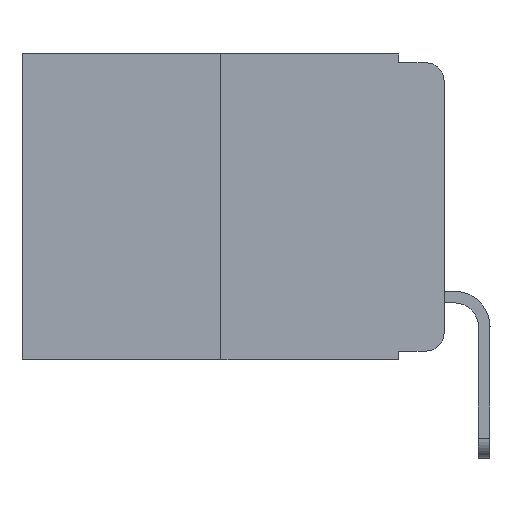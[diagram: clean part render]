
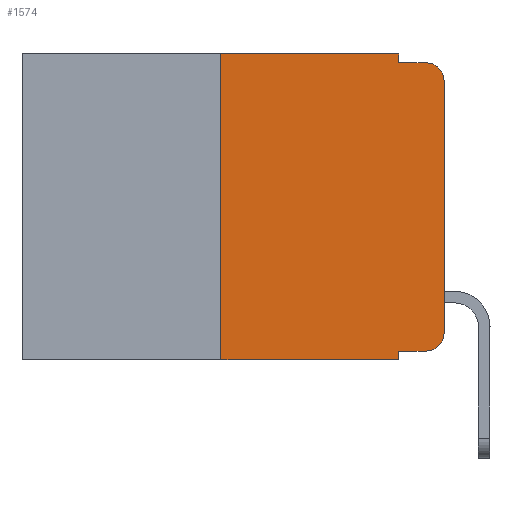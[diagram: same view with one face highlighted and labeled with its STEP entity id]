
A CAD part, left-side view. The second image highlights one B-rep face of the part: STEP entity #1574.
In plain terms, the highlighted planar face has unit normal (-1, 0, 0).
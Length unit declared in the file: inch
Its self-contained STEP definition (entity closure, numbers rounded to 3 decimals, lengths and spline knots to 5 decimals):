
#484 = CARTESIAN_POINT ( 'NONE',  ( 0., 0.25, 0. ) ) ;
#610 = EDGE_LOOP ( 'NONE', ( #824, #9862, #5833, #13297, #13022, #4682, #11914, #13391, #3550, #8004 ) ) ;
#616 = CARTESIAN_POINT ( 'NONE',  ( 0., 0., -0.313 ) ) ;
#824 = ORIENTED_EDGE ( 'NONE', *, *, #12422, .T. ) ;
#927 = VERTEX_POINT ( 'NONE', #6848 ) ;
#1211 = LINE ( 'NONE', #8619, #12267 ) ;
#1288 = EDGE_CURVE ( 'NONE', #4312, #3890, #7972, .T. ) ;
#1327 = DIRECTION ( 'NONE',  ( 0., -1., 0. ) ) ;
#1410 = CARTESIAN_POINT ( 'NONE',  ( 0., 0.051, -0.01 ) ) ;
#1574 = ADVANCED_FACE ( 'NONE', ( #6616 ), #6481, .F. ) ;
#1630 = DIRECTION ( 'NONE',  ( 0., -1., 0. ) ) ;
#1745 = DIRECTION ( 'NONE',  ( 0., -1., 0. ) ) ;
#2268 = DIRECTION ( 'NONE',  ( -1., 0., 0. ) ) ;
#2373 = VERTEX_POINT ( 'NONE', #616 ) ;
#2387 = LINE ( 'NONE', #8797, #4918 ) ;
#2411 = AXIS2_PLACEMENT_3D ( 'NONE', #8838, #7982, #7907 ) ;
#2805 = AXIS2_PLACEMENT_3D ( 'NONE', #11818, #2268, #8746 ) ;
#2826 = CARTESIAN_POINT ( 'NONE',  ( 0., 0.473, 0. ) ) ;
#2977 = VECTOR ( 'NONE', #11652, 39.37008 ) ;
#3105 = LINE ( 'NONE', #11745, #5889 ) ;
#3157 = VERTEX_POINT ( 'NONE', #8513 ) ;
#3550 = ORIENTED_EDGE ( 'NONE', *, *, #8214, .T. ) ;
#3738 = EDGE_CURVE ( 'NONE', #6555, #2373, #12442, .T. ) ;
#3823 = LINE ( 'NONE', #8264, #9161 ) ;
#3890 = VERTEX_POINT ( 'NONE', #7125 ) ;
#4067 = CARTESIAN_POINT ( 'NONE',  ( 0., 0., -0.03 ) ) ;
#4140 = EDGE_CURVE ( 'NONE', #7694, #6399, #5588, .T. ) ;
#4312 = VERTEX_POINT ( 'NONE', #4067 ) ;
#4591 = DIRECTION ( 'NONE',  ( 0., 0., 1. ) ) ;
#4682 = ORIENTED_EDGE ( 'NONE', *, *, #4140, .F. ) ;
#4714 = VECTOR ( 'NONE', #1745, 39.37008 ) ;
#4891 = DIRECTION ( 'NONE',  ( 0., 0., -1. ) ) ;
#4918 = VECTOR ( 'NONE', #1327, 39.37008 ) ;
#5342 = LINE ( 'NONE', #8439, #2977 ) ;
#5368 = CARTESIAN_POINT ( 'NONE',  ( 0., 0.02, -0.333 ) ) ;
#5435 = DIRECTION ( 'NONE',  ( 1., 0., 0. ) ) ;
#5523 = DIRECTION ( 'NONE',  ( 0., 0., -1. ) ) ;
#5588 = LINE ( 'NONE', #484, #13322 ) ;
#5833 = ORIENTED_EDGE ( 'NONE', *, *, #10413, .F. ) ;
#5889 = VECTOR ( 'NONE', #7387, 39.37008 ) ;
#5971 = EDGE_CURVE ( 'NONE', #3157, #12062, #3823, .T. ) ;
#6377 = VERTEX_POINT ( 'NONE', #1410 ) ;
#6399 = VERTEX_POINT ( 'NONE', #12319 ) ;
#6410 = CARTESIAN_POINT ( 'NONE',  ( 0., 0.051, -0.343 ) ) ;
#6416 = DIRECTION ( 'NONE',  ( 0., 0., -1. ) ) ;
#6481 = PLANE ( 'NONE',  #7869 ) ;
#6555 = VERTEX_POINT ( 'NONE', #5368 ) ;
#6616 = FACE_OUTER_BOUND ( 'NONE', #610, .T. ) ;
#6716 = EDGE_CURVE ( 'NONE', #7694, #12062, #2387, .T. ) ;
#6848 = CARTESIAN_POINT ( 'NONE',  ( 0., 0.051, 0. ) ) ;
#7046 = LINE ( 'NONE', #2826, #13811 ) ;
#7125 = CARTESIAN_POINT ( 'NONE',  ( 0., 0.02, -0.01 ) ) ;
#7387 = DIRECTION ( 'NONE',  ( 0., -1., 0. ) ) ;
#7403 = EDGE_CURVE ( 'NONE', #927, #6377, #1211, .T. ) ;
#7694 = VERTEX_POINT ( 'NONE', #8252 ) ;
#7721 = EDGE_CURVE ( 'NONE', #6399, #927, #7046, .T. ) ;
#7869 = AXIS2_PLACEMENT_3D ( 'NONE', #10721, #5435, #6416 ) ;
#7907 = DIRECTION ( 'NONE',  ( 0., 0., -1. ) ) ;
#7972 = CIRCLE ( 'NONE', #2805, 0.02 ) ;
#7982 = DIRECTION ( 'NONE',  ( -1., 0., 0. ) ) ;
#8004 = ORIENTED_EDGE ( 'NONE', *, *, #3738, .T. ) ;
#8214 = EDGE_CURVE ( 'NONE', #3157, #6555, #13263, .T. ) ;
#8252 = CARTESIAN_POINT ( 'NONE',  ( 0., 0.25, -0.343 ) ) ;
#8264 = CARTESIAN_POINT ( 'NONE',  ( 0., 0.051, 0. ) ) ;
#8439 = CARTESIAN_POINT ( 'NONE',  ( 0., 0., 0. ) ) ;
#8513 = CARTESIAN_POINT ( 'NONE',  ( 0., 0.051, -0.333 ) ) ;
#8619 = CARTESIAN_POINT ( 'NONE',  ( 0., 0.051, 0. ) ) ;
#8746 = DIRECTION ( 'NONE',  ( 0., 0., -1. ) ) ;
#8797 = CARTESIAN_POINT ( 'NONE',  ( 0., 0.473, -0.343 ) ) ;
#8838 = CARTESIAN_POINT ( 'NONE',  ( 0., 0.02, -0.313 ) ) ;
#9161 = VECTOR ( 'NONE', #4891, 39.37008 ) ;
#9862 = ORIENTED_EDGE ( 'NONE', *, *, #1288, .T. ) ;
#10413 = EDGE_CURVE ( 'NONE', #6377, #3890, #3105, .T. ) ;
#10721 = CARTESIAN_POINT ( 'NONE',  ( 0., 0.473, 0. ) ) ;
#11652 = DIRECTION ( 'NONE',  ( 0., 0., 1. ) ) ;
#11745 = CARTESIAN_POINT ( 'NONE',  ( 0., 0.051, -0.01 ) ) ;
#11818 = CARTESIAN_POINT ( 'NONE',  ( 0., 0.02, -0.03 ) ) ;
#11914 = ORIENTED_EDGE ( 'NONE', *, *, #6716, .T. ) ;
#12062 = VERTEX_POINT ( 'NONE', #6410 ) ;
#12267 = VECTOR ( 'NONE', #5523, 39.37008 ) ;
#12319 = CARTESIAN_POINT ( 'NONE',  ( 0., 0.25, 0. ) ) ;
#12422 = EDGE_CURVE ( 'NONE', #2373, #4312, #5342, .T. ) ;
#12442 = CIRCLE ( 'NONE', #2411, 0.02 ) ;
#12444 = CARTESIAN_POINT ( 'NONE',  ( 0., 0.051, -0.333 ) ) ;
#13022 = ORIENTED_EDGE ( 'NONE', *, *, #7721, .F. ) ;
#13263 = LINE ( 'NONE', #12444, #4714 ) ;
#13297 = ORIENTED_EDGE ( 'NONE', *, *, #7403, .F. ) ;
#13322 = VECTOR ( 'NONE', #4591, 39.37008 ) ;
#13391 = ORIENTED_EDGE ( 'NONE', *, *, #5971, .F. ) ;
#13811 = VECTOR ( 'NONE', #1630, 39.37008 ) ;
